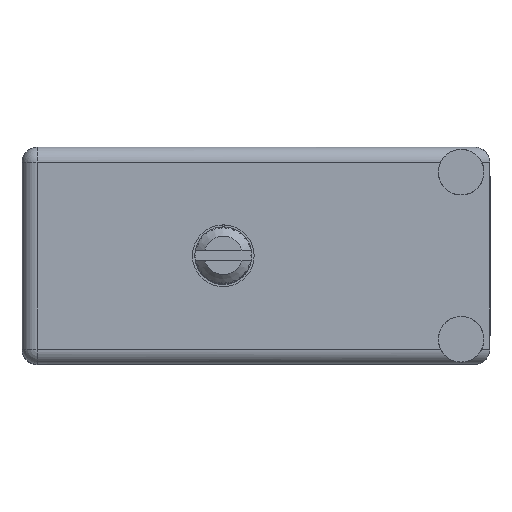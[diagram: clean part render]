
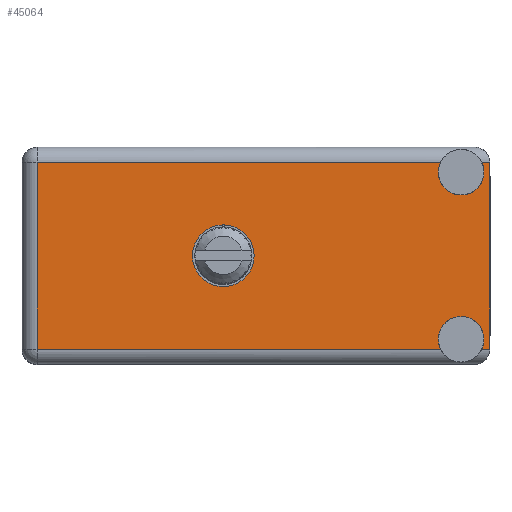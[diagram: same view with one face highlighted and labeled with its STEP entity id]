
A CAD part, top view. The second image highlights one B-rep face of the part: STEP entity #45064.
In plain terms, the highlighted face is planar.
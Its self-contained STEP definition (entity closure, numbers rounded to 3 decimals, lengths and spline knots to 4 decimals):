
#428 = EDGE_CURVE ( 'NONE', #115831, #84029, #59602, .T. ) ;
#1688 = ORIENTED_EDGE ( 'NONE', *, *, #5588, .F. ) ;
#4866 = ORIENTED_EDGE ( 'NONE', *, *, #162539, .T. ) ;
#5272 = CARTESIAN_POINT ( 'NONE',  ( 0., 0.806, 0. ) ) ;
#5588 = EDGE_CURVE ( 'NONE', #20097, #105596, #159787, .T. ) ;
#8377 = EDGE_CURVE ( 'NONE', #88165, #109725, #177910, .T. ) ;
#10984 = VECTOR ( 'NONE', #103188, 39.3701 ) ;
#12612 = CARTESIAN_POINT ( 'NONE',  ( 0.8501, 0.806, -0.3075 ) ) ;
#14148 = ORIENTED_EDGE ( 'NONE', *, *, #20378, .F. ) ;
#15285 = AXIS2_PLACEMENT_3D ( 'NONE', #175459, #44024, #58713 ) ;
#17490 = CIRCLE ( 'NONE', #38501, 0.075 ) ;
#20097 = VERTEX_POINT ( 'NONE', #54104 ) ;
#20378 = EDGE_CURVE ( 'NONE', #105596, #148515, #132488, .T. ) ;
#20413 = EDGE_CURVE ( 'NONE', #115831, #20728, #144124, .T. ) ;
#20728 = VERTEX_POINT ( 'NONE', #44297 ) ;
#26195 = DIRECTION ( 'NONE',  ( 0., 0., 1. ) ) ;
#28265 = CARTESIAN_POINT ( 'NONE',  ( 0.8765, 0.806, -0.3075 ) ) ;
#28568 = VERTEX_POINT ( 'NONE', #12612 ) ;
#31318 = VERTEX_POINT ( 'NONE', #28265 ) ;
#31911 = CARTESIAN_POINT ( 'NONE',  ( 0.8765, 0.806, 0.3575 ) ) ;
#32854 = CARTESIAN_POINT ( 'NONE',  ( 0.8765, 0.806, 0.3075 ) ) ;
#34322 = VECTOR ( 'NONE', #48520, 39.3701 ) ;
#37788 = ORIENTED_EDGE ( 'NONE', *, *, #90466, .T. ) ;
#38501 = AXIS2_PLACEMENT_3D ( 'NONE', #137916, #76958, #151460 ) ;
#40042 = CARTESIAN_POINT ( 'NONE',  ( 0.7825, 0.806, 0.2 ) ) ;
#40364 = DIRECTION ( 'NONE',  ( 0., 1., 0. ) ) ;
#44024 = DIRECTION ( 'NONE',  ( 0., 1., 0. ) ) ;
#44297 = CARTESIAN_POINT ( 'NONE',  ( -0.6125, 0.806, -0.3075 ) ) ;
#45064 = ADVANCED_FACE ( 'NONE', ( #97045, #94656 ), #58694, .T. ) ;
#48199 = ORIENTED_EDGE ( 'NONE', *, *, #122044, .T. ) ;
#48520 = DIRECTION ( 'NONE',  ( 1., 0., 0. ) ) ;
#49064 = DIRECTION ( 'NONE',  ( 1., 0., 0. ) ) ;
#54104 = CARTESIAN_POINT ( 'NONE',  ( 0.8501, 0.806, 0.3075 ) ) ;
#57183 = EDGE_CURVE ( 'NONE', #84029, #28568, #17490, .T. ) ;
#58694 = PLANE ( 'NONE',  #114582 ) ;
#58708 = CARTESIAN_POINT ( 'NONE',  ( 0.7149, 0.806, 0.3075 ) ) ;
#58713 = DIRECTION ( 'NONE',  ( 0., 0., 1. ) ) ;
#59602 = CIRCLE ( 'NONE', #91824, 0.075 ) ;
#61498 = VECTOR ( 'NONE', #188264, 39.3701 ) ;
#61589 = DIRECTION ( 'NONE',  ( 0., 0., 1. ) ) ;
#63169 = CARTESIAN_POINT ( 'NONE',  ( 0., 0.806, 0.1015 ) ) ;
#64335 = AXIS2_PLACEMENT_3D ( 'NONE', #5272, #166113, #61589 ) ;
#66369 = VECTOR ( 'NONE', #113950, 39.3701 ) ;
#70155 = CARTESIAN_POINT ( 'NONE',  ( 0.7825, 0.806, 0.275 ) ) ;
#70667 = LINE ( 'NONE', #166419, #144148 ) ;
#70782 = DIRECTION ( 'NONE',  ( 0., 1., 0. ) ) ;
#74721 = DIRECTION ( 'NONE',  ( 0., 0., 1. ) ) ;
#75945 = CARTESIAN_POINT ( 'NONE',  ( 0.7825, 0.806, -0.2 ) ) ;
#76958 = DIRECTION ( 'NONE',  ( 0., 1., 0. ) ) ;
#82288 = LINE ( 'NONE', #82534, #66369 ) ;
#82534 = CARTESIAN_POINT ( 'NONE',  ( -0.6625, 0.806, -0.3075 ) ) ;
#83839 = DIRECTION ( 'NONE',  ( 0., 0., 1. ) ) ;
#84029 = VERTEX_POINT ( 'NONE', #75945 ) ;
#84274 = ORIENTED_EDGE ( 'NONE', *, *, #428, .F. ) ;
#88165 = VERTEX_POINT ( 'NONE', #182444 ) ;
#89386 = DIRECTION ( 'NONE',  ( -1., 0., 0. ) ) ;
#90466 = EDGE_CURVE ( 'NONE', #116172, #148515, #112320, .T. ) ;
#91316 = DIRECTION ( 'NONE',  ( 0., 1., 0. ) ) ;
#91824 = AXIS2_PLACEMENT_3D ( 'NONE', #171806, #40364, #83839 ) ;
#92366 = EDGE_CURVE ( 'NONE', #20097, #143474, #70667, .T. ) ;
#94656 = FACE_OUTER_BOUND ( 'NONE', #143156, .T. ) ;
#97045 = FACE_BOUND ( 'NONE', #165848, .T. ) ;
#103118 = EDGE_CURVE ( 'NONE', #109725, #88165, #183856, .T. ) ;
#103188 = DIRECTION ( 'NONE',  ( 0., 0., 1. ) ) ;
#105596 = VERTEX_POINT ( 'NONE', #40042 ) ;
#106752 = ORIENTED_EDGE ( 'NONE', *, *, #8377, .F. ) ;
#109363 = LINE ( 'NONE', #31911, #111548 ) ;
#109725 = VERTEX_POINT ( 'NONE', #63169 ) ;
#111548 = VECTOR ( 'NONE', #74721, 39.3701 ) ;
#112320 = LINE ( 'NONE', #136346, #34322 ) ;
#113950 = DIRECTION ( 'NONE',  ( -1., 0., 0. ) ) ;
#114582 = AXIS2_PLACEMENT_3D ( 'NONE', #147198, #91316, #89386 ) ;
#115831 = VERTEX_POINT ( 'NONE', #138493 ) ;
#116172 = VERTEX_POINT ( 'NONE', #175842 ) ;
#119859 = ORIENTED_EDGE ( 'NONE', *, *, #57183, .F. ) ;
#119882 = ORIENTED_EDGE ( 'NONE', *, *, #103118, .F. ) ;
#120177 = ORIENTED_EDGE ( 'NONE', *, *, #164188, .F. ) ;
#122044 = EDGE_CURVE ( 'NONE', #31318, #28568, #82288, .T. ) ;
#132488 = CIRCLE ( 'NONE', #155980, 0.075 ) ;
#136346 = CARTESIAN_POINT ( 'NONE',  ( 0.8765, 0.806, 0.3075 ) ) ;
#137916 = CARTESIAN_POINT ( 'NONE',  ( 0.7825, 0.806, -0.275 ) ) ;
#138493 = CARTESIAN_POINT ( 'NONE',  ( 0.7149, 0.806, -0.3075 ) ) ;
#143156 = EDGE_LOOP ( 'NONE', ( #37788, #14148, #1688, #143755, #120177, #48199, #119859, #84274, #181787, #4866 ) ) ;
#143474 = VERTEX_POINT ( 'NONE', #32854 ) ;
#143755 = ORIENTED_EDGE ( 'NONE', *, *, #92366, .T. ) ;
#144124 = LINE ( 'NONE', #173445, #61498 ) ;
#144148 = VECTOR ( 'NONE', #49064, 39.3701 ) ;
#147198 = CARTESIAN_POINT ( 'NONE',  ( -0.6625, 0.806, -0.3575 ) ) ;
#147216 = AXIS2_PLACEMENT_3D ( 'NONE', #158280, #158905, #26195 ) ;
#148515 = VERTEX_POINT ( 'NONE', #58708 ) ;
#151460 = DIRECTION ( 'NONE',  ( 0., 0., 1. ) ) ;
#155980 = AXIS2_PLACEMENT_3D ( 'NONE', #70155, #70782, #172809 ) ;
#158280 = CARTESIAN_POINT ( 'NONE',  ( 0., 0.806, 0. ) ) ;
#158905 = DIRECTION ( 'NONE',  ( 0., 1., 0. ) ) ;
#159787 = CIRCLE ( 'NONE', #15285, 0.075 ) ;
#162305 = CARTESIAN_POINT ( 'NONE',  ( -0.6125, 0.806, -0.3575 ) ) ;
#162539 = EDGE_CURVE ( 'NONE', #20728, #116172, #190011, .T. ) ;
#164188 = EDGE_CURVE ( 'NONE', #31318, #143474, #109363, .T. ) ;
#165848 = EDGE_LOOP ( 'NONE', ( #119882, #106752 ) ) ;
#166113 = DIRECTION ( 'NONE',  ( 0., 1., 0. ) ) ;
#166419 = CARTESIAN_POINT ( 'NONE',  ( 0.8765, 0.806, 0.3075 ) ) ;
#171806 = CARTESIAN_POINT ( 'NONE',  ( 0.7825, 0.806, -0.275 ) ) ;
#172809 = DIRECTION ( 'NONE',  ( 0., 0., 1. ) ) ;
#173445 = CARTESIAN_POINT ( 'NONE',  ( -0.6625, 0.806, -0.3075 ) ) ;
#175459 = CARTESIAN_POINT ( 'NONE',  ( 0.7825, 0.806, 0.275 ) ) ;
#175842 = CARTESIAN_POINT ( 'NONE',  ( -0.6125, 0.806, 0.3075 ) ) ;
#177910 = CIRCLE ( 'NONE', #147216, 0.1015 ) ;
#181787 = ORIENTED_EDGE ( 'NONE', *, *, #20413, .T. ) ;
#182444 = CARTESIAN_POINT ( 'NONE',  ( 0., 0.806, -0.1015 ) ) ;
#183856 = CIRCLE ( 'NONE', #64335, 0.1015 ) ;
#188264 = DIRECTION ( 'NONE',  ( -1., 0., 0. ) ) ;
#190011 = LINE ( 'NONE', #162305, #10984 ) ;
